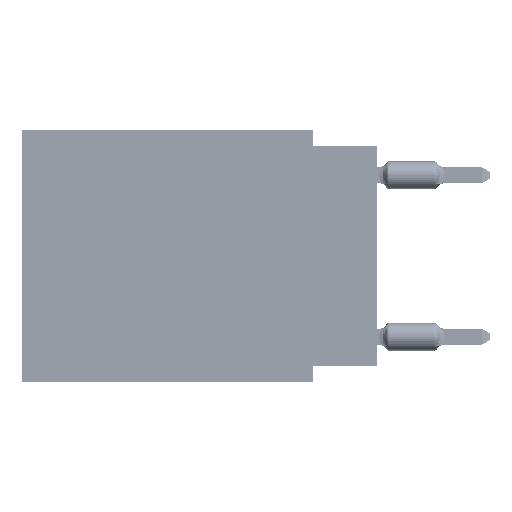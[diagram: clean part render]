
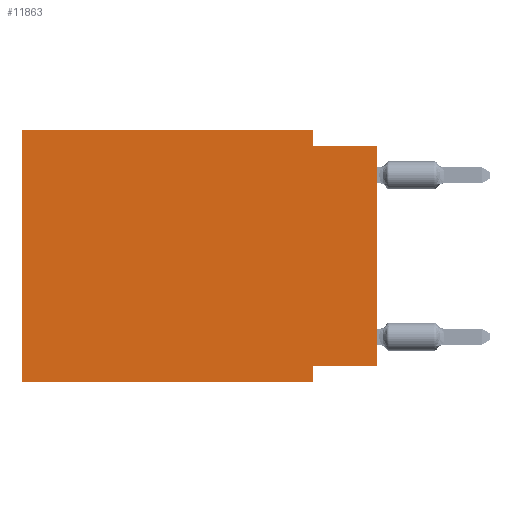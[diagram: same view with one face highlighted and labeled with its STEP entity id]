
A CAD part, left-side view. The second image highlights one B-rep face of the part: STEP entity #11863.
In plain terms, the highlighted planar face has unit normal (-1, 0, 0).
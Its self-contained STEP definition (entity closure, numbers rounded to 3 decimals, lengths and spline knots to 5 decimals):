
#183 = EDGE_CURVE ( 'NONE', #73828, #13751, #36195, .T. ) ;
#3252 = LINE ( 'NONE', #22076, #40665 ) ;
#4961 = DIRECTION ( 'NONE',  ( 0., 0., -1. ) ) ;
#5027 = VECTOR ( 'NONE', #28260, 39.37008 ) ;
#5991 = CARTESIAN_POINT ( 'NONE',  ( 0., 0.1, -0.39 ) ) ;
#11357 = DIRECTION ( 'NONE',  ( 0., -1., 0. ) ) ;
#11863 = ADVANCED_FACE ( 'NONE', ( #24761 ), #44417, .F. ) ;
#13751 = VERTEX_POINT ( 'NONE', #5991 ) ;
#14879 = CARTESIAN_POINT ( 'NONE',  ( 0., 0.1, -0.39 ) ) ;
#15068 = LINE ( 'NONE', #41131, #65803 ) ;
#15750 = EDGE_CURVE ( 'NONE', #52030, #84127, #31024, .T. ) ;
#18057 = EDGE_CURVE ( 'NONE', #22977, #28696, #3252, .T. ) ;
#18549 = EDGE_CURVE ( 'NONE', #22977, #73828, #81227, .T. ) ;
#20554 = CARTESIAN_POINT ( 'NONE',  ( 0., 0.1, 0. ) ) ;
#22076 = CARTESIAN_POINT ( 'NONE',  ( 0., 0., 0. ) ) ;
#22977 = VERTEX_POINT ( 'NONE', #67172 ) ;
#24761 = FACE_OUTER_BOUND ( 'NONE', #60589, .T. ) ;
#25025 = CARTESIAN_POINT ( 'NONE',  ( 0., 0., -0.025 ) ) ;
#27434 = ORIENTED_EDGE ( 'NONE', *, *, #18057, .T. ) ;
#27781 = CARTESIAN_POINT ( 'NONE',  ( 0., 0.1, -0.025 ) ) ;
#27914 = CARTESIAN_POINT ( 'NONE',  ( 0., 0.55, 0. ) ) ;
#28260 = DIRECTION ( 'NONE',  ( 0., 1., 0. ) ) ;
#28696 = VERTEX_POINT ( 'NONE', #49626 ) ;
#31024 = LINE ( 'NONE', #71181, #45903 ) ;
#31764 = EDGE_CURVE ( 'NONE', #84127, #28696, #63911, .T. ) ;
#32003 = DIRECTION ( 'NONE',  ( 0., 0., -1. ) ) ;
#32951 = ORIENTED_EDGE ( 'NONE', *, *, #46661, .F. ) ;
#33388 = EDGE_CURVE ( 'NONE', #42837, #78467, #66817, .T. ) ;
#36195 = LINE ( 'NONE', #14879, #41352 ) ;
#36871 = ORIENTED_EDGE ( 'NONE', *, *, #72046, .T. ) ;
#38746 = ORIENTED_EDGE ( 'NONE', *, *, #18549, .F. ) ;
#38961 = DIRECTION ( 'NONE',  ( 0., -1., 0. ) ) ;
#40304 = DIRECTION ( 'NONE',  ( 0., 0., 1. ) ) ;
#40665 = VECTOR ( 'NONE', #41739, 39.37008 ) ;
#41131 = CARTESIAN_POINT ( 'NONE',  ( 0., 0.55, -0.39 ) ) ;
#41352 = VECTOR ( 'NONE', #53782, 39.37008 ) ;
#41739 = DIRECTION ( 'NONE',  ( 0., 0., 1. ) ) ;
#42121 = CARTESIAN_POINT ( 'NONE',  ( 0., 0.55, -0.39 ) ) ;
#42837 = VERTEX_POINT ( 'NONE', #42121 ) ;
#44417 = PLANE ( 'NONE',  #68698 ) ;
#44434 = VECTOR ( 'NONE', #38961, 39.37008 ) ;
#45392 = LINE ( 'NONE', #71457, #44434 ) ;
#45903 = VECTOR ( 'NONE', #4961, 39.37008 ) ;
#46661 = EDGE_CURVE ( 'NONE', #78467, #52030, #45392, .T. ) ;
#49188 = CARTESIAN_POINT ( 'NONE',  ( 0., 0., -0.365 ) ) ;
#49626 = CARTESIAN_POINT ( 'NONE',  ( 0., 0., -0.025 ) ) ;
#50438 = VECTOR ( 'NONE', #11357, 39.37008 ) ;
#52030 = VERTEX_POINT ( 'NONE', #20554 ) ;
#53782 = DIRECTION ( 'NONE',  ( 0., 0., -1. ) ) ;
#55088 = ORIENTED_EDGE ( 'NONE', *, *, #183, .F. ) ;
#58380 = VECTOR ( 'NONE', #40304, 39.37008 ) ;
#60589 = EDGE_LOOP ( 'NONE', ( #27434, #81857, #70470, #32951, #79124, #36871, #55088, #38746 ) ) ;
#63911 = LINE ( 'NONE', #25025, #50438 ) ;
#65803 = VECTOR ( 'NONE', #67203, 39.37008 ) ;
#66817 = LINE ( 'NONE', #27914, #58380 ) ;
#67172 = CARTESIAN_POINT ( 'NONE',  ( 0., 0., -0.365 ) ) ;
#67203 = DIRECTION ( 'NONE',  ( 0., -1., 0. ) ) ;
#68698 = AXIS2_PLACEMENT_3D ( 'NONE', #71325, #70900, #32003 ) ;
#69930 = CARTESIAN_POINT ( 'NONE',  ( 0., 0.55, 0. ) ) ;
#70470 = ORIENTED_EDGE ( 'NONE', *, *, #15750, .F. ) ;
#70900 = DIRECTION ( 'NONE',  ( 1., 0., 0. ) ) ;
#71181 = CARTESIAN_POINT ( 'NONE',  ( 0., 0.1, 0. ) ) ;
#71325 = CARTESIAN_POINT ( 'NONE',  ( 0., 0.55, 0. ) ) ;
#71457 = CARTESIAN_POINT ( 'NONE',  ( 0., 0.55, 0. ) ) ;
#72046 = EDGE_CURVE ( 'NONE', #42837, #13751, #15068, .T. ) ;
#73828 = VERTEX_POINT ( 'NONE', #73903 ) ;
#73903 = CARTESIAN_POINT ( 'NONE',  ( 0., 0.1, -0.365 ) ) ;
#78467 = VERTEX_POINT ( 'NONE', #69930 ) ;
#79124 = ORIENTED_EDGE ( 'NONE', *, *, #33388, .F. ) ;
#81227 = LINE ( 'NONE', #49188, #5027 ) ;
#81857 = ORIENTED_EDGE ( 'NONE', *, *, #31764, .F. ) ;
#84127 = VERTEX_POINT ( 'NONE', #27781 ) ;
